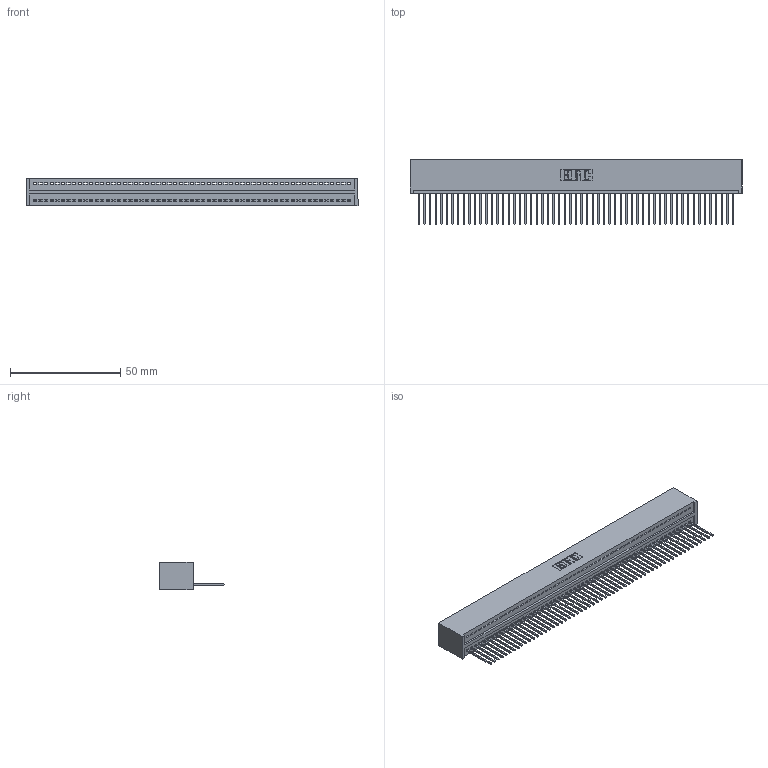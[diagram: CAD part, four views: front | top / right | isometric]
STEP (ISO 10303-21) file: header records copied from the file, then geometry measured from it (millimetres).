
FILE_DESCRIPTION (( 'STEP AP203' ), '1' );
FILE_NAME ('325-057-540-101.STEP', '2020-02-25T01:45:20', ( '' ), ( '' ), 'SwSTEP 2.0', 'SolidWorks 2016', '' );
FILE_SCHEMA (( 'CONFIG_CONTROL_DESIGN' ));
Length unit declared in the file: inch
Products named in the file (3): 325 Part_Lugless; 325-292-001_325-293-140; 325-057-540-101
Assembly tree (58 placements, depth 2):
  325-057-540-101
    325 Part_Lugless
    325-292-001_325-293-140  x57
Bounding box: 150.42 x 29.46 x 12.45 mm (x, y, z)
Volume: 19862.7 mm3; surface area: 23015.8 mm2
Topology: 58 solids, 58 shells, 3412 faces, 10319 edges, 6802 vertices
Faces by surface type: plane 2460, cylinder 952
Entity records: 32647 total; most frequent: CARTESIAN_POINT 5637, ORIENTED_EDGE 5630, DIRECTION 4717, EDGE_CURVE 2815, LINE 2695, VECTOR 2695, VERTEX_POINT 1874, AXIS2_PLACEMENT_3D 1011
